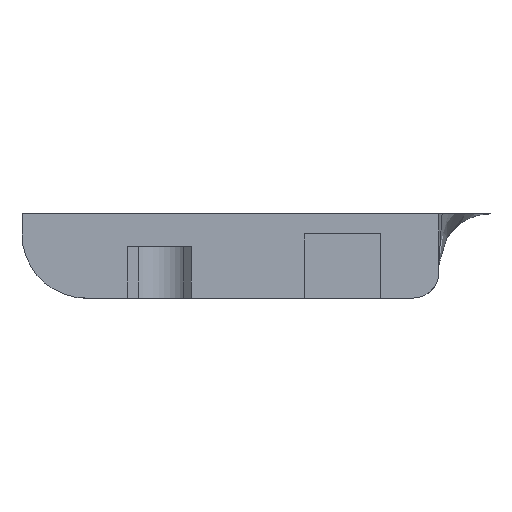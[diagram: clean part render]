
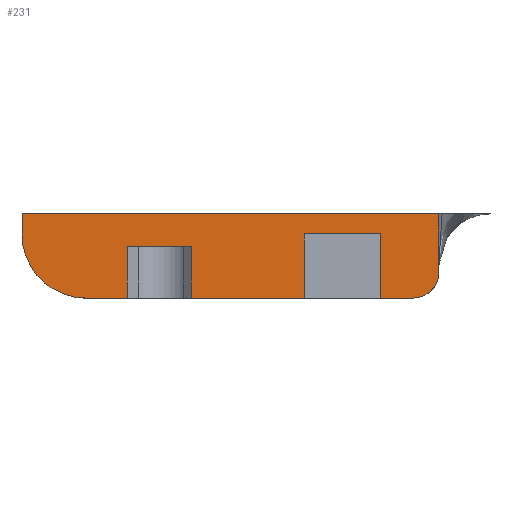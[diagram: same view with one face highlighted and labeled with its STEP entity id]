
A CAD part, left-side view. The second image highlights one B-rep face of the part: STEP entity #231.
In plain terms, the highlighted planar face has unit normal (-1, 0, 0).
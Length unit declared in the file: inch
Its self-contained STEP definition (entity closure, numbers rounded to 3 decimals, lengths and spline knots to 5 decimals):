
#8 = DIRECTION ( 'NONE',  ( 1., 0., 0. ) ) ;
#14 = AXIS2_PLACEMENT_3D ( 'NONE', #473, #8, #1060 ) ;
#22 = VERTEX_POINT ( 'NONE', #941 ) ;
#25 = EDGE_CURVE ( 'NONE', #200, #626, #1253, .T. ) ;
#36 = ORIENTED_EDGE ( 'NONE', *, *, #1698, .T. ) ;
#58 = ORIENTED_EDGE ( 'NONE', *, *, #1822, .F. ) ;
#60 = CARTESIAN_POINT ( 'NONE',  ( 3.70038, 1.32551, -0.47244 ) ) ;
#68 = CARTESIAN_POINT ( 'NONE',  ( 3.70038, -1.79442, -1.11943 ) ) ;
#88 = ORIENTED_EDGE ( 'NONE', *, *, #1598, .F. ) ;
#98 = VECTOR ( 'NONE', #971, 39.37008 ) ;
#99 = CARTESIAN_POINT ( 'NONE',  ( 3.70038, -0.71157, -0.73097 ) ) ;
#135 = CARTESIAN_POINT ( 'NONE',  ( 3.70038, -1.79442, -0.47244 ) ) ;
#141 = CARTESIAN_POINT ( 'NONE',  ( 3.70038, -0.51472, -0.70907 ) ) ;
#147 = CARTESIAN_POINT ( 'NONE',  ( 3.70038, -0.83807, -0.53412 ) ) ;
#148 = EDGE_CURVE ( 'NONE', #1894, #1080, #1284, .T. ) ;
#149 = LINE ( 'NONE', #833, #98 ) ;
#200 = VERTEX_POINT ( 'NONE', #1821 ) ;
#225 = CIRCLE ( 'NONE', #422, 0.19685 ) ;
#229 = DIRECTION ( 'NONE',  ( 0., 0., -1. ) ) ;
#231 = ADVANCED_FACE ( 'NONE', ( #1952 ), #775, .F. ) ;
#246 = DIRECTION ( 'NONE',  ( 0., 1., 0. ) ) ;
#340 = VERTEX_POINT ( 'NONE', #987 ) ;
#349 = DIRECTION ( 'NONE',  ( 0., 1., 0. ) ) ;
#376 = CARTESIAN_POINT ( 'NONE',  ( 3.70038, -1.38086, -0.73097 ) ) ;
#377 = AXIS2_PLACEMENT_3D ( 'NONE', #526, #1555, #678 ) ;
#420 = LINE ( 'NONE', #141, #469 ) ;
#422 = AXIS2_PLACEMENT_3D ( 'NONE', #1375, #493, #1522 ) ;
#426 = CARTESIAN_POINT ( 'NONE',  ( 3.70038, -1.79442, -0.62992 ) ) ;
#432 = EDGE_CURVE ( 'NONE', #1213, #873, #1564, .T. ) ;
#467 = VECTOR ( 'NONE', #1425, 39.37008 ) ;
#469 = VECTOR ( 'NONE', #1040, 39.37008 ) ;
#473 = CARTESIAN_POINT ( 'NONE',  ( 3.70038, 1.01705, 0.74273 ) ) ;
#493 = DIRECTION ( 'NONE',  ( -1., 0., 0. ) ) ;
#497 = CARTESIAN_POINT ( 'NONE',  ( 3.70038, -1.38086, -0.53412 ) ) ;
#511 = CARTESIAN_POINT ( 'NONE',  ( 3.70038, -0.51472, -0.53412 ) ) ;
#518 = LINE ( 'NONE', #68, #1248 ) ;
#526 = CARTESIAN_POINT ( 'NONE',  ( 3.70038, -1.71568, -0.65223 ) ) ;
#533 = CARTESIAN_POINT ( 'NONE',  ( 3.70038, -0.47716, -0.73097 ) ) ;
#539 = DIRECTION ( 'NONE',  ( 0., 0., -1. ) ) ;
#575 = VECTOR ( 'NONE', #1264, 39.37008 ) ;
#621 = LINE ( 'NONE', #533, #661 ) ;
#626 = VERTEX_POINT ( 'NONE', #1606 ) ;
#634 = ORIENTED_EDGE ( 'NONE', *, *, #148, .F. ) ;
#659 = VERTEX_POINT ( 'NONE', #99 ) ;
#661 = VECTOR ( 'NONE', #961, 39.37008 ) ;
#678 = DIRECTION ( 'NONE',  ( 0., 1., 0. ) ) ;
#684 = DIRECTION ( 'NONE',  ( 0., -1., 0. ) ) ;
#692 = DIRECTION ( 'NONE',  ( 0., 1., 0. ) ) ;
#727 = CARTESIAN_POINT ( 'NONE',  ( 3.70038, -1.03493, -0.73097 ) ) ;
#747 = ORIENTED_EDGE ( 'NONE', *, *, #1819, .F. ) ;
#755 = CARTESIAN_POINT ( 'NONE',  ( 3.70038, -1.03493, -0.57349 ) ) ;
#760 = VERTEX_POINT ( 'NONE', #426 ) ;
#768 = DIRECTION ( 'NONE',  ( 0., 0., -1. ) ) ;
#775 = PLANE ( 'NONE',  #14 ) ;
#782 = VECTOR ( 'NONE', #1568, 39.37008 ) ;
#827 = CARTESIAN_POINT ( 'NONE',  ( 3.70038, -0.8125, -0.57349 ) ) ;
#833 = CARTESIAN_POINT ( 'NONE',  ( 3.70038, -1.61708, 0. ) ) ;
#873 = VERTEX_POINT ( 'NONE', #135 ) ;
#913 = VECTOR ( 'NONE', #692, 39.37008 ) ;
#941 = CARTESIAN_POINT ( 'NONE',  ( 3.70038, -1.61708, -0.53412 ) ) ;
#946 = VERTEX_POINT ( 'NONE', #497 ) ;
#948 = LINE ( 'NONE', #376, #1705 ) ;
#958 = ORIENTED_EDGE ( 'NONE', *, *, #1760, .T. ) ;
#961 = DIRECTION ( 'NONE',  ( 0., 1., 0. ) ) ;
#971 = DIRECTION ( 'NONE',  ( 0., 0., -1. ) ) ;
#987 = CARTESIAN_POINT ( 'NONE',  ( 3.70038, -1.79442, -0.65223 ) ) ;
#998 = LINE ( 'NONE', #827, #1351 ) ;
#1040 = DIRECTION ( 'NONE',  ( 0., 0., 1. ) ) ;
#1045 = LINE ( 'NONE', #1115, #575 ) ;
#1060 = DIRECTION ( 'NONE',  ( 0., 1., 0. ) ) ;
#1072 = VERTEX_POINT ( 'NONE', #511 ) ;
#1080 = VERTEX_POINT ( 'NONE', #1236 ) ;
#1083 = VECTOR ( 'NONE', #246, 39.37008 ) ;
#1115 = CARTESIAN_POINT ( 'NONE',  ( 3.70038, -1.03493, -0.53412 ) ) ;
#1129 = CARTESIAN_POINT ( 'NONE',  ( 3.70038, -0.51472, -0.47244 ) ) ;
#1132 = CARTESIAN_POINT ( 'NONE',  ( 3.70038, -0.47716, -0.73097 ) ) ;
#1173 = ORIENTED_EDGE ( 'NONE', *, *, #1438, .F. ) ;
#1194 = EDGE_LOOP ( 'NONE', ( #1897, #88, #36, #1817, #634, #1316, #1666, #1173, #1935, #747, #1479, #1832, #958, #58, #1809 ) ) ;
#1207 = VECTOR ( 'NONE', #349, 39.37008 ) ;
#1213 = VERTEX_POINT ( 'NONE', #1129 ) ;
#1227 = VECTOR ( 'NONE', #768, 39.37008 ) ;
#1236 = CARTESIAN_POINT ( 'NONE',  ( 3.70038, -0.83807, -0.73097 ) ) ;
#1239 = CARTESIAN_POINT ( 'NONE',  ( 3.70038, -0.83807, -0.57349 ) ) ;
#1248 = VECTOR ( 'NONE', #229, 39.37008 ) ;
#1253 = LINE ( 'NONE', #1381, #1207 ) ;
#1264 = DIRECTION ( 'NONE',  ( 0., 0., 1. ) ) ;
#1271 = CARTESIAN_POINT ( 'NONE',  ( 3.70038, -1.79442, -1.63124 ) ) ;
#1284 = LINE ( 'NONE', #147, #1227 ) ;
#1316 = ORIENTED_EDGE ( 'NONE', *, *, #1801, .T. ) ;
#1351 = VECTOR ( 'NONE', #684, 39.37008 ) ;
#1375 = CARTESIAN_POINT ( 'NONE',  ( 3.70038, -0.71157, -0.53412 ) ) ;
#1381 = CARTESIAN_POINT ( 'NONE',  ( 3.70038, -0.47716, -0.73097 ) ) ;
#1394 = VERTEX_POINT ( 'NONE', #1882 ) ;
#1425 = DIRECTION ( 'NONE',  ( 0., 0., 1. ) ) ;
#1438 = EDGE_CURVE ( 'NONE', #1394, #1495, #1492, .T. ) ;
#1479 = ORIENTED_EDGE ( 'NONE', *, *, #1820, .T. ) ;
#1492 = LINE ( 'NONE', #1132, #1083 ) ;
#1495 = VERTEX_POINT ( 'NONE', #727 ) ;
#1522 = DIRECTION ( 'NONE',  ( 0., 1., 0. ) ) ;
#1555 = DIRECTION ( 'NONE',  ( -1., 0., 0. ) ) ;
#1564 = LINE ( 'NONE', #60, #782 ) ;
#1568 = DIRECTION ( 'NONE',  ( 0., -1., 0. ) ) ;
#1570 = CARTESIAN_POINT ( 'NONE',  ( 3.70038, -1.38086, -0.53412 ) ) ;
#1585 = VERTEX_POINT ( 'NONE', #755 ) ;
#1598 = EDGE_CURVE ( 'NONE', #1072, #1213, #420, .T. ) ;
#1606 = CARTESIAN_POINT ( 'NONE',  ( 3.70038, -1.61708, -0.73097 ) ) ;
#1655 = LINE ( 'NONE', #1271, #467 ) ;
#1666 = ORIENTED_EDGE ( 'NONE', *, *, #1803, .F. ) ;
#1698 = EDGE_CURVE ( 'NONE', #1072, #659, #225, .T. ) ;
#1705 = VECTOR ( 'NONE', #539, 39.37008 ) ;
#1760 = EDGE_CURVE ( 'NONE', #200, #340, #1844, .T. ) ;
#1762 = LINE ( 'NONE', #1570, #913 ) ;
#1788 = EDGE_CURVE ( 'NONE', #1080, #659, #621, .T. ) ;
#1801 = EDGE_CURVE ( 'NONE', #1894, #1585, #998, .T. ) ;
#1803 = EDGE_CURVE ( 'NONE', #1495, #1585, #1045, .T. ) ;
#1808 = EDGE_CURVE ( 'NONE', #946, #1394, #948, .T. ) ;
#1809 = ORIENTED_EDGE ( 'NONE', *, *, #1828, .T. ) ;
#1817 = ORIENTED_EDGE ( 'NONE', *, *, #1788, .F. ) ;
#1819 = EDGE_CURVE ( 'NONE', #22, #946, #1762, .T. ) ;
#1820 = EDGE_CURVE ( 'NONE', #22, #626, #149, .T. ) ;
#1821 = CARTESIAN_POINT ( 'NONE',  ( 3.70038, -1.71568, -0.73097 ) ) ;
#1822 = EDGE_CURVE ( 'NONE', #760, #340, #518, .T. ) ;
#1828 = EDGE_CURVE ( 'NONE', #760, #873, #1655, .T. ) ;
#1832 = ORIENTED_EDGE ( 'NONE', *, *, #25, .F. ) ;
#1844 = CIRCLE ( 'NONE', #377, 0.07874 ) ;
#1882 = CARTESIAN_POINT ( 'NONE',  ( 3.70038, -1.38086, -0.73097 ) ) ;
#1894 = VERTEX_POINT ( 'NONE', #1239 ) ;
#1897 = ORIENTED_EDGE ( 'NONE', *, *, #432, .F. ) ;
#1935 = ORIENTED_EDGE ( 'NONE', *, *, #1808, .F. ) ;
#1952 = FACE_OUTER_BOUND ( 'NONE', #1194, .T. ) ;
